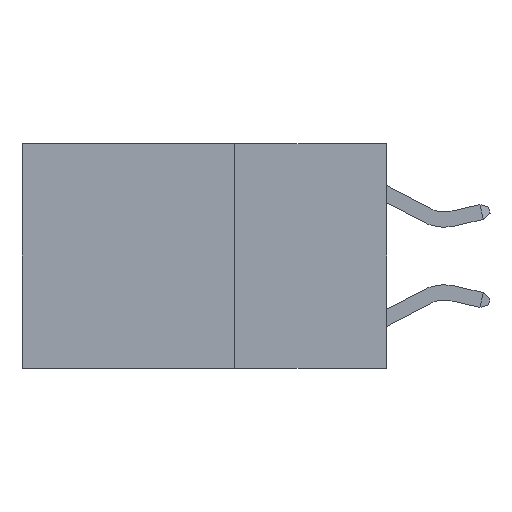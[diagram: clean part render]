
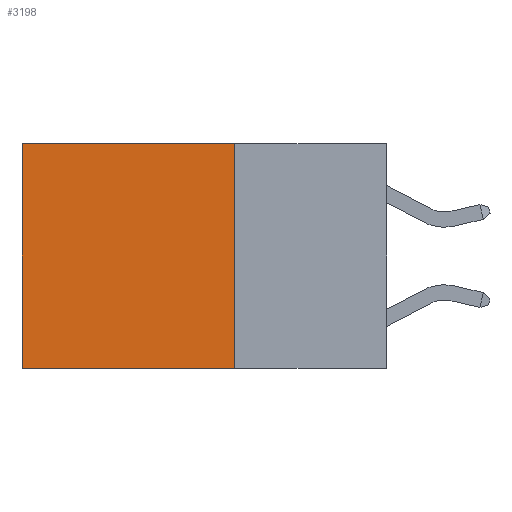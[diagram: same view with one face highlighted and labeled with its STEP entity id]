
A CAD part, left-side view. The second image highlights one B-rep face of the part: STEP entity #3198.
In plain terms, the highlighted planar face has unit normal (-1, 0, 0).
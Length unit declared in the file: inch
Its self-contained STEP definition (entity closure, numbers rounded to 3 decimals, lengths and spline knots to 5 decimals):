
#567 = CARTESIAN_POINT ( 'NONE',  ( 0.2625, 0.25, 0. ) ) ;
#959 = CARTESIAN_POINT ( 'NONE',  ( 0.2625, 0.25, 0. ) ) ;
#1873 = VECTOR ( 'NONE', #2885, 39.37008 ) ;
#2100 = VECTOR ( 'NONE', #13052, 39.37008 ) ;
#2651 = CARTESIAN_POINT ( 'NONE',  ( 0.2625, 0.6, 0. ) ) ;
#2885 = DIRECTION ( 'NONE',  ( 0., 0., -1. ) ) ;
#3011 = VERTEX_POINT ( 'NONE', #14449 ) ;
#3198 = ADVANCED_FACE ( 'NONE', ( #16794 ), #16896, .F. ) ;
#3272 = CARTESIAN_POINT ( 'NONE',  ( 0.2625, 0.25, 0. ) ) ;
#4581 = DIRECTION ( 'NONE',  ( 0., 0., -1. ) ) ;
#4704 = LINE ( 'NONE', #567, #9280 ) ;
#5291 = EDGE_CURVE ( 'NONE', #3011, #13275, #7220, .T. ) ;
#7163 = DIRECTION ( 'NONE',  ( 0., 0., -1. ) ) ;
#7220 = LINE ( 'NONE', #22630, #2100 ) ;
#7999 = EDGE_CURVE ( 'NONE', #17310, #18017, #4704, .T. ) ;
#9215 = ORIENTED_EDGE ( 'NONE', *, *, #5291, .F. ) ;
#9280 = VECTOR ( 'NONE', #10255, 39.37008 ) ;
#9551 = EDGE_LOOP ( 'NONE', ( #24033, #9215, #11744, #13430 ) ) ;
#10255 = DIRECTION ( 'NONE',  ( 0., 1., 0. ) ) ;
#11744 = ORIENTED_EDGE ( 'NONE', *, *, #24905, .F. ) ;
#13052 = DIRECTION ( 'NONE',  ( 0., 1., 0. ) ) ;
#13275 = VERTEX_POINT ( 'NONE', #24268 ) ;
#13430 = ORIENTED_EDGE ( 'NONE', *, *, #7999, .T. ) ;
#13676 = EDGE_CURVE ( 'NONE', #18017, #13275, #19258, .T. ) ;
#14449 = CARTESIAN_POINT ( 'NONE',  ( 0.2625, 0.25, -0.37 ) ) ;
#15251 = AXIS2_PLACEMENT_3D ( 'NONE', #3272, #18825, #7163 ) ;
#16794 = FACE_OUTER_BOUND ( 'NONE', #9551, .T. ) ;
#16896 = PLANE ( 'NONE',  #15251 ) ;
#17310 = VERTEX_POINT ( 'NONE', #24243 ) ;
#17451 = VECTOR ( 'NONE', #4581, 39.37008 ) ;
#18017 = VERTEX_POINT ( 'NONE', #18644 ) ;
#18644 = CARTESIAN_POINT ( 'NONE',  ( 0.2625, 0.6, 0. ) ) ;
#18825 = DIRECTION ( 'NONE',  ( 1., 0., 0. ) ) ;
#19258 = LINE ( 'NONE', #2651, #17451 ) ;
#22519 = LINE ( 'NONE', #959, #1873 ) ;
#22630 = CARTESIAN_POINT ( 'NONE',  ( 0.2625, 0.25, -0.37 ) ) ;
#24033 = ORIENTED_EDGE ( 'NONE', *, *, #13676, .T. ) ;
#24243 = CARTESIAN_POINT ( 'NONE',  ( 0.2625, 0.25, 0. ) ) ;
#24268 = CARTESIAN_POINT ( 'NONE',  ( 0.2625, 0.6, -0.37 ) ) ;
#24905 = EDGE_CURVE ( 'NONE', #17310, #3011, #22519, .T. ) ;
